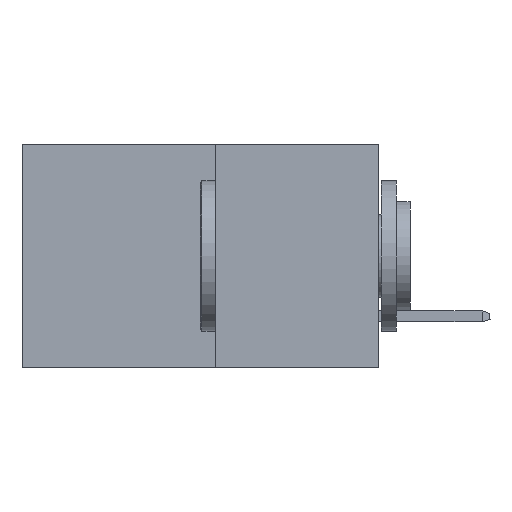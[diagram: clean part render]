
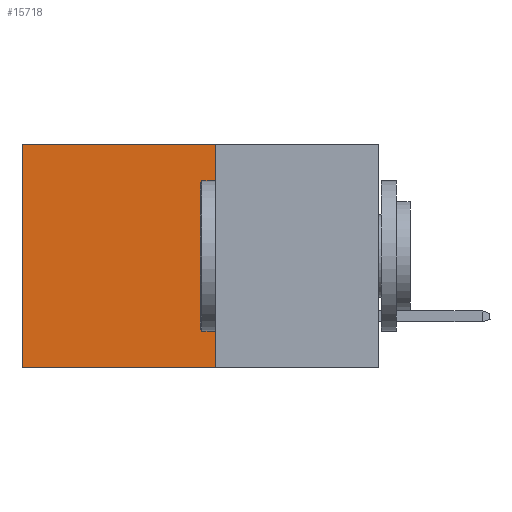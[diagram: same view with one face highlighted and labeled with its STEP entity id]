
A CAD part, left-side view. The second image highlights one B-rep face of the part: STEP entity #15718.
In plain terms, the highlighted planar face has unit normal (-1, 0, 0).
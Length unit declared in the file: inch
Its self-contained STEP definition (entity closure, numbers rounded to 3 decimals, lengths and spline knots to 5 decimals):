
#63 = DIRECTION ( 'NONE',  ( 1., 0., 0. ) ) ;
#318 = ORIENTED_EDGE ( 'NONE', *, *, #18086, .T. ) ;
#2803 = EDGE_CURVE ( 'NONE', #5039, #8698, #6876, .T. ) ;
#2903 = CARTESIAN_POINT ( 'NONE',  ( 0.277, 0.59, -0.37 ) ) ;
#2965 = CARTESIAN_POINT ( 'NONE',  ( 0.277, 0.59, 0. ) ) ;
#3185 = CARTESIAN_POINT ( 'NONE',  ( 0.277, 0.27, 0. ) ) ;
#3645 = VECTOR ( 'NONE', #11303, 39.37008 ) ;
#4313 = PLANE ( 'NONE',  #10186 ) ;
#5039 = VERTEX_POINT ( 'NONE', #10090 ) ;
#6544 = ORIENTED_EDGE ( 'NONE', *, *, #2803, .F. ) ;
#6764 = CARTESIAN_POINT ( 'NONE',  ( 0.277, 0.27, -0.37 ) ) ;
#6876 = LINE ( 'NONE', #13848, #14748 ) ;
#8061 = EDGE_LOOP ( 'NONE', ( #14656, #16935, #6544, #318 ) ) ;
#8284 = EDGE_CURVE ( 'NONE', #8698, #12708, #17971, .T. ) ;
#8611 = FACE_OUTER_BOUND ( 'NONE', #8061, .T. ) ;
#8698 = VERTEX_POINT ( 'NONE', #6764 ) ;
#9977 = DIRECTION ( 'NONE',  ( 0., 0., -1. ) ) ;
#10090 = CARTESIAN_POINT ( 'NONE',  ( 0.277, 0.27, 0. ) ) ;
#10186 = AXIS2_PLACEMENT_3D ( 'NONE', #16860, #63, #9977 ) ;
#10679 = VECTOR ( 'NONE', #13648, 39.37008 ) ;
#10724 = VECTOR ( 'NONE', #12982, 39.37008 ) ;
#11104 = LINE ( 'NONE', #2903, #3645 ) ;
#11303 = DIRECTION ( 'NONE',  ( 0., 0., -1. ) ) ;
#12105 = EDGE_CURVE ( 'NONE', #12164, #12708, #11104, .T. ) ;
#12164 = VERTEX_POINT ( 'NONE', #2965 ) ;
#12236 = CARTESIAN_POINT ( 'NONE',  ( 0.277, 0.27, -0.37 ) ) ;
#12699 = CARTESIAN_POINT ( 'NONE',  ( 0.277, 0.59, -0.37 ) ) ;
#12708 = VERTEX_POINT ( 'NONE', #12699 ) ;
#12982 = DIRECTION ( 'NONE',  ( 0., 1., 0. ) ) ;
#13648 = DIRECTION ( 'NONE',  ( 0., 1., 0. ) ) ;
#13819 = DIRECTION ( 'NONE',  ( 0., 0., -1. ) ) ;
#13848 = CARTESIAN_POINT ( 'NONE',  ( 0.277, 0.27, -0.37 ) ) ;
#14436 = LINE ( 'NONE', #3185, #10724 ) ;
#14656 = ORIENTED_EDGE ( 'NONE', *, *, #12105, .T. ) ;
#14748 = VECTOR ( 'NONE', #13819, 39.37008 ) ;
#15718 = ADVANCED_FACE ( 'NONE', ( #8611 ), #4313, .F. ) ;
#16860 = CARTESIAN_POINT ( 'NONE',  ( 0.277, 0.27, -0.37 ) ) ;
#16935 = ORIENTED_EDGE ( 'NONE', *, *, #8284, .F. ) ;
#17971 = LINE ( 'NONE', #12236, #10679 ) ;
#18086 = EDGE_CURVE ( 'NONE', #5039, #12164, #14436, .T. ) ;
